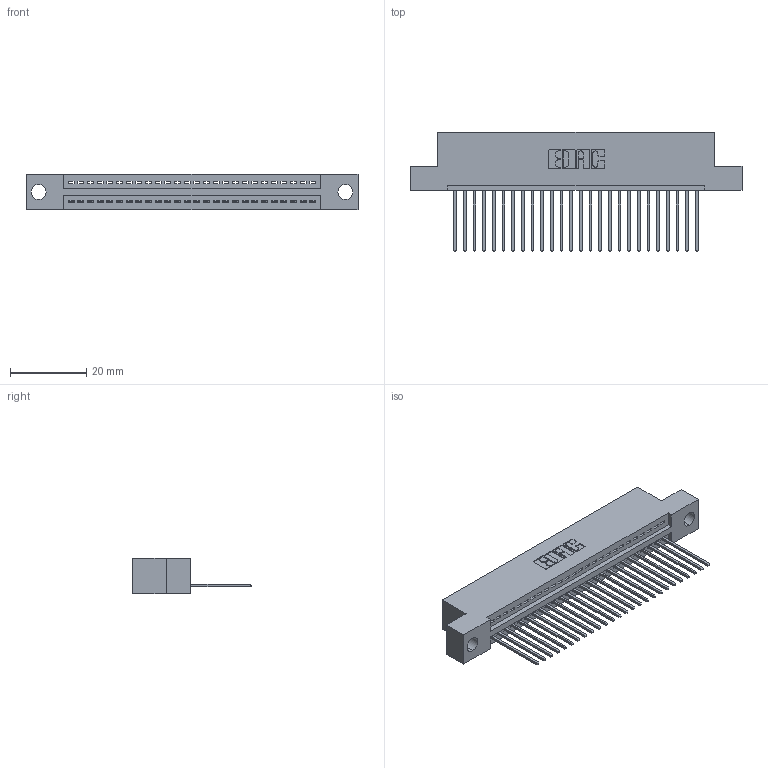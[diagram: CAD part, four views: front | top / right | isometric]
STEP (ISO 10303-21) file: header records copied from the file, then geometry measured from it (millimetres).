
FILE_DESCRIPTION (( 'STEP AP203' ), '1' );
FILE_NAME ('395-026-542-104.STEP', '2021-05-31T14:38:03', ( '' ), ( '' ), 'SwSTEP 2.0', 'SolidWorks 2020', '' );
FILE_SCHEMA (( 'CONFIG_CONTROL_DESIGN' ));
Length unit declared in the file: inch
Products named in the file (3): 395-026-542-104; 345 Part_Flush Mounting Lugs - 0.156 Dia-TI; 345-292-001_345-293-142
Assembly tree (27 placements, depth 2):
  395-026-542-104
    345 Part_Flush Mounting Lugs - 0.156 Dia-TI
    345-292-001_345-293-142  x26
Bounding box: 87.25 x 31.29 x 9.4 mm (x, y, z)
Volume: 8107.8 mm3; surface area: 10765.4 mm2
Topology: 27 solids, 27 shells, 1648 faces, 4953 edges, 3266 vertices
Faces by surface type: plane 1134, cylinder 514
Entity records: 22159 total; most frequent: CARTESIAN_POINT 3848, ORIENTED_EDGE 3806, DIRECTION 3383, EDGE_CURVE 1903, LINE 1667, VECTOR 1667, VERTEX_POINT 1266, AXIS2_PLACEMENT_3D 858
